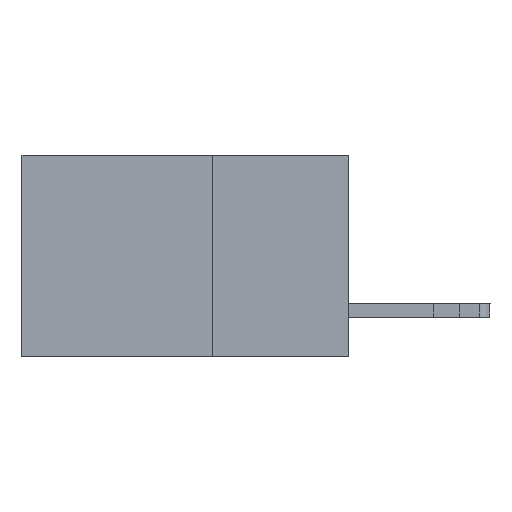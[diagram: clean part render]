
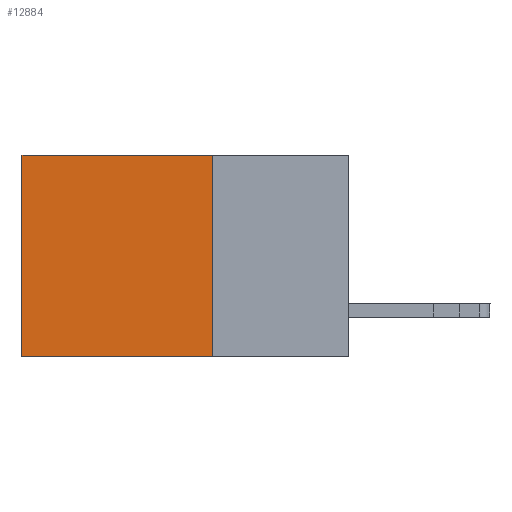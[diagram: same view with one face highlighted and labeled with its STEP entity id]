
A CAD part, left-side view. The second image highlights one B-rep face of the part: STEP entity #12884.
In plain terms, the highlighted planar face has unit normal (-1, 0, 0).
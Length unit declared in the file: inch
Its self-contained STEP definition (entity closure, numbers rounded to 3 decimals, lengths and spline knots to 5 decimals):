
#1023 = CARTESIAN_POINT ( 'NONE',  ( 0.298, 0.25, 0. ) ) ;
#1100 = ORIENTED_EDGE ( 'NONE', *, *, #10497, .T. ) ;
#1955 = CARTESIAN_POINT ( 'NONE',  ( 0.298, 0.6, 0. ) ) ;
#2234 = EDGE_CURVE ( 'NONE', #10488, #16441, #15775, .T. ) ;
#3526 = CARTESIAN_POINT ( 'NONE',  ( 0.298, 0.25, 0. ) ) ;
#5376 = EDGE_CURVE ( 'NONE', #16441, #16678, #11839, .T. ) ;
#6374 = CARTESIAN_POINT ( 'NONE',  ( 0.298, 0.6, 0. ) ) ;
#6724 = AXIS2_PLACEMENT_3D ( 'NONE', #12320, #6951, #9377 ) ;
#6811 = DIRECTION ( 'NONE',  ( 0., 0., -1. ) ) ;
#6951 = DIRECTION ( 'NONE',  ( 1., 0., 0. ) ) ;
#7816 = CARTESIAN_POINT ( 'NONE',  ( 0.298, 0.25, -0.37 ) ) ;
#8053 = VECTOR ( 'NONE', #6811, 39.37008 ) ;
#8568 = VERTEX_POINT ( 'NONE', #1955 ) ;
#8872 = LINE ( 'NONE', #6374, #15779 ) ;
#9377 = DIRECTION ( 'NONE',  ( 0., 0., -1. ) ) ;
#9634 = PLANE ( 'NONE',  #6724 ) ;
#10449 = EDGE_CURVE ( 'NONE', #8568, #16678, #8872, .T. ) ;
#10488 = VERTEX_POINT ( 'NONE', #1023 ) ;
#10497 = EDGE_CURVE ( 'NONE', #10488, #8568, #14303, .T. ) ;
#10645 = DIRECTION ( 'NONE',  ( 0., 1., 0. ) ) ;
#11588 = ORIENTED_EDGE ( 'NONE', *, *, #2234, .F. ) ;
#11839 = LINE ( 'NONE', #14511, #15500 ) ;
#11983 = FACE_OUTER_BOUND ( 'NONE', #17023, .T. ) ;
#12320 = CARTESIAN_POINT ( 'NONE',  ( 0.298, 0.25, 0. ) ) ;
#12884 = ADVANCED_FACE ( 'NONE', ( #11983 ), #9634, .F. ) ;
#12886 = ORIENTED_EDGE ( 'NONE', *, *, #5376, .F. ) ;
#13111 = DIRECTION ( 'NONE',  ( 0., 1., 0. ) ) ;
#13315 = ORIENTED_EDGE ( 'NONE', *, *, #10449, .T. ) ;
#14128 = VECTOR ( 'NONE', #13111, 39.37008 ) ;
#14303 = LINE ( 'NONE', #3526, #14128 ) ;
#14490 = CARTESIAN_POINT ( 'NONE',  ( 0.298, 0.25, 0. ) ) ;
#14511 = CARTESIAN_POINT ( 'NONE',  ( 0.298, 0.25, -0.37 ) ) ;
#15211 = CARTESIAN_POINT ( 'NONE',  ( 0.298, 0.6, -0.37 ) ) ;
#15500 = VECTOR ( 'NONE', #10645, 39.37008 ) ;
#15518 = DIRECTION ( 'NONE',  ( 0., 0., -1. ) ) ;
#15775 = LINE ( 'NONE', #14490, #8053 ) ;
#15779 = VECTOR ( 'NONE', #15518, 39.37008 ) ;
#16441 = VERTEX_POINT ( 'NONE', #7816 ) ;
#16678 = VERTEX_POINT ( 'NONE', #15211 ) ;
#17023 = EDGE_LOOP ( 'NONE', ( #13315, #12886, #11588, #1100 ) ) ;
